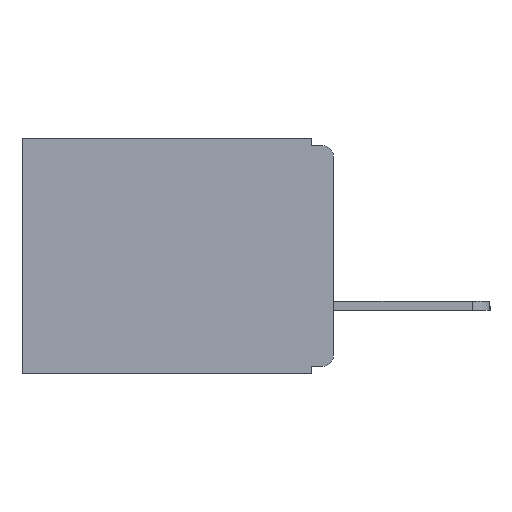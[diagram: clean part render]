
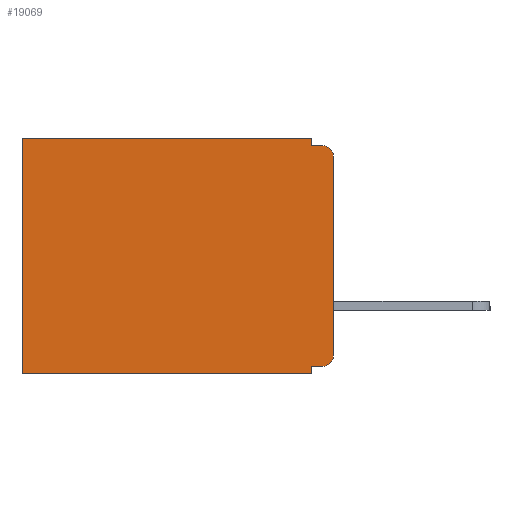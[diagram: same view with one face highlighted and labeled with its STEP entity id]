
A CAD part, left-side view. The second image highlights one B-rep face of the part: STEP entity #19069.
In plain terms, the highlighted planar face has unit normal (-1, 0, 0).
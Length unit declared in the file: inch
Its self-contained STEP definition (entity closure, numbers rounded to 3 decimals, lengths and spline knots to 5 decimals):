
#197 = CARTESIAN_POINT ( 'NONE',  ( 0.3, 0.015, -0.305 ) ) ;
#944 = EDGE_CURVE ( 'NONE', #9294, #7419, #16426, .T. ) ;
#1337 = LINE ( 'NONE', #4614, #5816 ) ;
#1366 = CARTESIAN_POINT ( 'NONE',  ( 0.3, 0., -0.025 ) ) ;
#1652 = LINE ( 'NONE', #8238, #9952 ) ;
#1841 = DIRECTION ( 'NONE',  ( 0., 0., -1. ) ) ;
#1936 = CARTESIAN_POINT ( 'NONE',  ( 0.3, 0.015, -0.32 ) ) ;
#1977 = VECTOR ( 'NONE', #5755, 39.37008 ) ;
#2021 = VERTEX_POINT ( 'NONE', #7195 ) ;
#3390 = ORIENTED_EDGE ( 'NONE', *, *, #18276, .F. ) ;
#3587 = VERTEX_POINT ( 'NONE', #12466 ) ;
#4614 = CARTESIAN_POINT ( 'NONE',  ( 0.3, 0., -0.01 ) ) ;
#4798 = VERTEX_POINT ( 'NONE', #1936 ) ;
#4943 = EDGE_CURVE ( 'NONE', #6670, #2021, #19989, .T. ) ;
#5147 = DIRECTION ( 'NONE',  ( 0., 0., -1. ) ) ;
#5252 = ORIENTED_EDGE ( 'NONE', *, *, #5679, .T. ) ;
#5428 = DIRECTION ( 'NONE',  ( 1., 0., 0. ) ) ;
#5643 = AXIS2_PLACEMENT_3D ( 'NONE', #15224, #5428, #16825 ) ;
#5679 = EDGE_CURVE ( 'NONE', #6670, #9016, #19716, .T. ) ;
#5736 = VERTEX_POINT ( 'NONE', #16126 ) ;
#5755 = DIRECTION ( 'NONE',  ( 0., 1., 0. ) ) ;
#5816 = VECTOR ( 'NONE', #17651, 39.37008 ) ;
#6048 = ORIENTED_EDGE ( 'NONE', *, *, #17136, .F. ) ;
#6217 = CARTESIAN_POINT ( 'NONE',  ( 0.3, 0.015, -0.025 ) ) ;
#6542 = CARTESIAN_POINT ( 'NONE',  ( 0.3, 0., -0.33 ) ) ;
#6670 = VERTEX_POINT ( 'NONE', #19931 ) ;
#6836 = EDGE_CURVE ( 'NONE', #9016, #3587, #14556, .T. ) ;
#6882 = DIRECTION ( 'NONE',  ( 0., 0., -1. ) ) ;
#7195 = CARTESIAN_POINT ( 'NONE',  ( 0.3, 0.031, -0.01 ) ) ;
#7264 = FACE_OUTER_BOUND ( 'NONE', #19714, .T. ) ;
#7419 = VERTEX_POINT ( 'NONE', #20836 ) ;
#7860 = DIRECTION ( 'NONE',  ( 0., 0., -1. ) ) ;
#8213 = DIRECTION ( 'NONE',  ( 0., 1., 0. ) ) ;
#8238 = CARTESIAN_POINT ( 'NONE',  ( 0.3, 0.031, -0.33 ) ) ;
#9016 = VERTEX_POINT ( 'NONE', #15501 ) ;
#9294 = VERTEX_POINT ( 'NONE', #1366 ) ;
#9467 = CIRCLE ( 'NONE', #17289, 0.015 ) ;
#9859 = DIRECTION ( 'NONE',  ( 0., 0., -1. ) ) ;
#9952 = VECTOR ( 'NONE', #9859, 39.37008 ) ;
#10215 = VECTOR ( 'NONE', #6882, 39.37008 ) ;
#11045 = EDGE_CURVE ( 'NONE', #9294, #5736, #13143, .T. ) ;
#11271 = VECTOR ( 'NONE', #11681, 39.37008 ) ;
#11305 = DIRECTION ( 'NONE',  ( 0., 0., -1. ) ) ;
#11562 = VECTOR ( 'NONE', #11305, 39.37008 ) ;
#11681 = DIRECTION ( 'NONE',  ( 0., 1., 0. ) ) ;
#11781 = DIRECTION ( 'NONE',  ( -1., 0., 0. ) ) ;
#12130 = AXIS2_PLACEMENT_3D ( 'NONE', #6217, #17552, #7860 ) ;
#12176 = LINE ( 'NONE', #6542, #20082 ) ;
#12466 = CARTESIAN_POINT ( 'NONE',  ( 0.3, 0.437, -0.33 ) ) ;
#12712 = ORIENTED_EDGE ( 'NONE', *, *, #4943, .F. ) ;
#13143 = CIRCLE ( 'NONE', #12130, 0.015 ) ;
#14011 = ORIENTED_EDGE ( 'NONE', *, *, #15029, .T. ) ;
#14556 = LINE ( 'NONE', #16151, #10215 ) ;
#15029 = EDGE_CURVE ( 'NONE', #4798, #7419, #9467, .T. ) ;
#15112 = CARTESIAN_POINT ( 'NONE',  ( 0.3, 0.031, 0. ) ) ;
#15224 = CARTESIAN_POINT ( 'NONE',  ( 0.3, 0., -0.33 ) ) ;
#15283 = ORIENTED_EDGE ( 'NONE', *, *, #16055, .F. ) ;
#15501 = CARTESIAN_POINT ( 'NONE',  ( 0.3, 0.437, 0. ) ) ;
#15529 = CARTESIAN_POINT ( 'NONE',  ( 0.3, 0., -0.32 ) ) ;
#15637 = LINE ( 'NONE', #15529, #1977 ) ;
#15693 = CARTESIAN_POINT ( 'NONE',  ( 0.3, 0.031, -0.32 ) ) ;
#15835 = VERTEX_POINT ( 'NONE', #18890 ) ;
#15972 = ORIENTED_EDGE ( 'NONE', *, *, #944, .F. ) ;
#16055 = EDGE_CURVE ( 'NONE', #19750, #15835, #1652, .T. ) ;
#16126 = CARTESIAN_POINT ( 'NONE',  ( 0.3, 0.015, -0.01 ) ) ;
#16151 = CARTESIAN_POINT ( 'NONE',  ( 0.3, 0.437, -0.33 ) ) ;
#16426 = LINE ( 'NONE', #17666, #20523 ) ;
#16825 = DIRECTION ( 'NONE',  ( 0., 0., -1. ) ) ;
#17136 = EDGE_CURVE ( 'NONE', #2021, #5736, #1337, .T. ) ;
#17228 = CARTESIAN_POINT ( 'NONE',  ( 0.3, 0., 0. ) ) ;
#17275 = ORIENTED_EDGE ( 'NONE', *, *, #20282, .F. ) ;
#17289 = AXIS2_PLACEMENT_3D ( 'NONE', #197, #11781, #1841 ) ;
#17552 = DIRECTION ( 'NONE',  ( -1., 0., 0. ) ) ;
#17651 = DIRECTION ( 'NONE',  ( 0., -1., 0. ) ) ;
#17666 = CARTESIAN_POINT ( 'NONE',  ( 0.3, 0., -0.33 ) ) ;
#17957 = ORIENTED_EDGE ( 'NONE', *, *, #11045, .T. ) ;
#18276 = EDGE_CURVE ( 'NONE', #15835, #3587, #12176, .T. ) ;
#18890 = CARTESIAN_POINT ( 'NONE',  ( 0.3, 0.031, -0.33 ) ) ;
#19069 = ADVANCED_FACE ( 'NONE', ( #7264 ), #19852, .F. ) ;
#19369 = ORIENTED_EDGE ( 'NONE', *, *, #6836, .T. ) ;
#19714 = EDGE_LOOP ( 'NONE', ( #15972, #17957, #6048, #12712, #5252, #19369, #3390, #15283, #17275, #14011 ) ) ;
#19716 = LINE ( 'NONE', #17228, #11271 ) ;
#19750 = VERTEX_POINT ( 'NONE', #15693 ) ;
#19852 = PLANE ( 'NONE',  #5643 ) ;
#19931 = CARTESIAN_POINT ( 'NONE',  ( 0.3, 0.031, 0. ) ) ;
#19989 = LINE ( 'NONE', #15112, #11562 ) ;
#20082 = VECTOR ( 'NONE', #8213, 39.37008 ) ;
#20282 = EDGE_CURVE ( 'NONE', #4798, #19750, #15637, .T. ) ;
#20523 = VECTOR ( 'NONE', #5147, 39.37008 ) ;
#20836 = CARTESIAN_POINT ( 'NONE',  ( 0.3, 0., -0.305 ) ) ;
